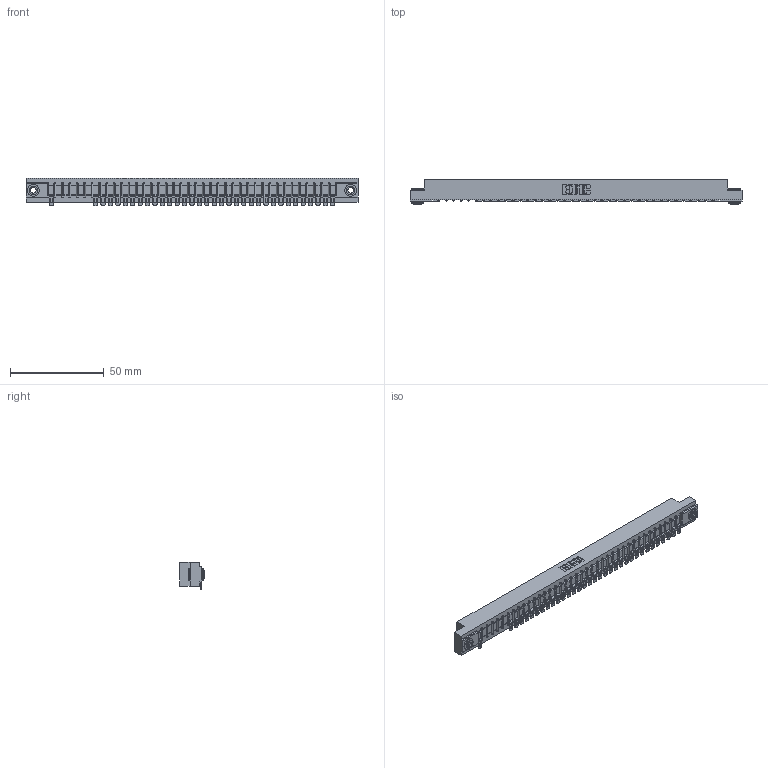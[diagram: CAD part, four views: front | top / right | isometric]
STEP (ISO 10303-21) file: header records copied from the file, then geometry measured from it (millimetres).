
FILE_DESCRIPTION (( 'STEP AP203' ), '1' );
FILE_NAME ('357-039-554-103.STEP', '2018-08-11T04:28:51', ( '' ), ( '' ), 'SwSTEP 2.0', 'SolidWorks 2016', '' );
FILE_SCHEMA (( 'CONFIG_CONTROL_DESIGN' ));
Length unit declared in the file: inch
Products named in the file (4): 307 Part_.156 Dia Mounting Holes; 307-290-002_554; 345-250-002_345-250-002-102; 357-039-554-103
Assembly tree (37 placements, depth 2):
  357-039-554-103
    307 Part_.156 Dia Mounting Holes
    307-290-002_554  x34
    345-250-002_345-250-002-102  x2
Bounding box: 177.55 x 13.36 x 14.52 mm (x, y, z)
Volume: 18846.2 mm3; surface area: 23084.1 mm2
Topology: 37 solids, 37 shells, 3064 faces, 9357 edges, 6126 vertices
Faces by surface type: plane 1718, cylinder 1258, sphere 80, cone 8
Entity records: 35674 total; most frequent: CARTESIAN_POINT 6018, ORIENTED_EDGE 6004, DIRECTION 5864, EDGE_CURVE 3002, VECTOR 2284, LINE 2284, VERTEX_POINT 1944, AXIS2_PLACEMENT_3D 1790
